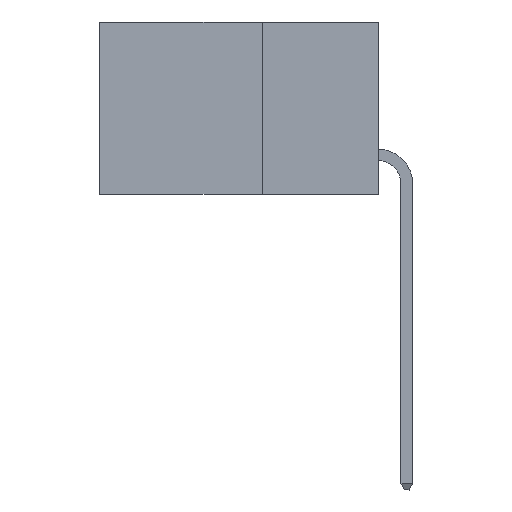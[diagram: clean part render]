
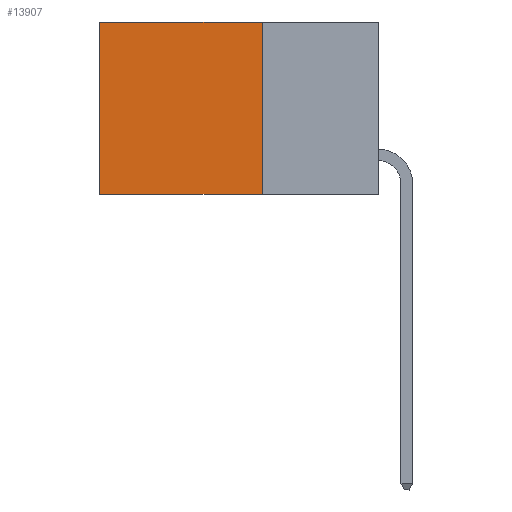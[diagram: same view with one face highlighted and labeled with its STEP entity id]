
A CAD part, left-side view. The second image highlights one B-rep face of the part: STEP entity #13907.
In plain terms, the highlighted planar face has unit normal (-1, 0, 0).
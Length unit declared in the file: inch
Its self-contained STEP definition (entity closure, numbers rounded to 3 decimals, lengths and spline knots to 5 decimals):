
#154 = CARTESIAN_POINT ( 'NONE',  ( 0.298, 0.25, -0.37 ) ) ;
#190 = VECTOR ( 'NONE', #3664, 39.37008 ) ;
#195 = VERTEX_POINT ( 'NONE', #10669 ) ;
#738 = VECTOR ( 'NONE', #3909, 39.37008 ) ;
#3003 = EDGE_CURVE ( 'NONE', #17214, #8709, #4224, .T. ) ;
#3112 = EDGE_CURVE ( 'NONE', #8959, #17214, #13769, .T. ) ;
#3236 = ORIENTED_EDGE ( 'NONE', *, *, #8371, .T. ) ;
#3571 = CARTESIAN_POINT ( 'NONE',  ( 0.298, 0.25, 0. ) ) ;
#3664 = DIRECTION ( 'NONE',  ( 0., 1., 0. ) ) ;
#3770 = CARTESIAN_POINT ( 'NONE',  ( 0.298, 0.25, 0. ) ) ;
#3824 = CARTESIAN_POINT ( 'NONE',  ( 0.298, 0.25, 0. ) ) ;
#3909 = DIRECTION ( 'NONE',  ( 0., 1., 0. ) ) ;
#4224 = LINE ( 'NONE', #154, #190 ) ;
#5033 = DIRECTION ( 'NONE',  ( 0., 0., -1. ) ) ;
#5459 = LINE ( 'NONE', #9575, #16174 ) ;
#5496 = AXIS2_PLACEMENT_3D ( 'NONE', #3571, #13539, #5033 ) ;
#5915 = CARTESIAN_POINT ( 'NONE',  ( 0.298, 0.25, 0. ) ) ;
#6586 = CARTESIAN_POINT ( 'NONE',  ( 0.298, 0.6, -0.37 ) ) ;
#7661 = DIRECTION ( 'NONE',  ( 0., 0., -1. ) ) ;
#8371 = EDGE_CURVE ( 'NONE', #195, #8709, #5459, .T. ) ;
#8709 = VERTEX_POINT ( 'NONE', #6586 ) ;
#8956 = EDGE_CURVE ( 'NONE', #8959, #195, #15518, .T. ) ;
#8959 = VERTEX_POINT ( 'NONE', #3770 ) ;
#9483 = DIRECTION ( 'NONE',  ( 0., 0., -1. ) ) ;
#9575 = CARTESIAN_POINT ( 'NONE',  ( 0.298, 0.6, 0. ) ) ;
#10084 = VECTOR ( 'NONE', #7661, 39.37008 ) ;
#10669 = CARTESIAN_POINT ( 'NONE',  ( 0.298, 0.6, 0. ) ) ;
#10756 = PLANE ( 'NONE',  #5496 ) ;
#10984 = CARTESIAN_POINT ( 'NONE',  ( 0.298, 0.25, -0.37 ) ) ;
#11877 = ORIENTED_EDGE ( 'NONE', *, *, #3003, .F. ) ;
#12400 = FACE_OUTER_BOUND ( 'NONE', #14927, .T. ) ;
#13539 = DIRECTION ( 'NONE',  ( 1., 0., 0. ) ) ;
#13769 = LINE ( 'NONE', #5915, #10084 ) ;
#13907 = ADVANCED_FACE ( 'NONE', ( #12400 ), #10756, .F. ) ;
#14619 = ORIENTED_EDGE ( 'NONE', *, *, #8956, .T. ) ;
#14927 = EDGE_LOOP ( 'NONE', ( #3236, #11877, #14965, #14619 ) ) ;
#14965 = ORIENTED_EDGE ( 'NONE', *, *, #3112, .F. ) ;
#15518 = LINE ( 'NONE', #3824, #738 ) ;
#16174 = VECTOR ( 'NONE', #9483, 39.37008 ) ;
#17214 = VERTEX_POINT ( 'NONE', #10984 ) ;
